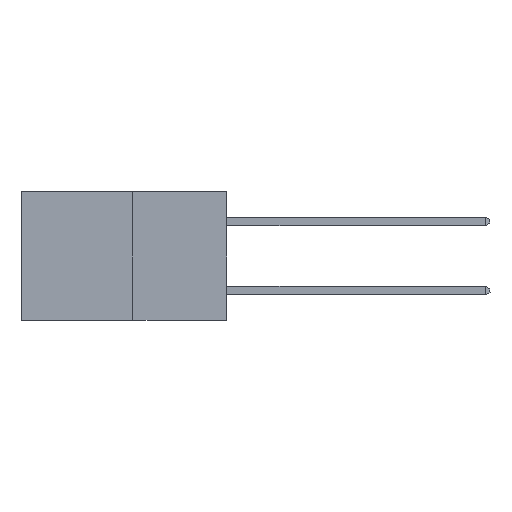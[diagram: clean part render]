
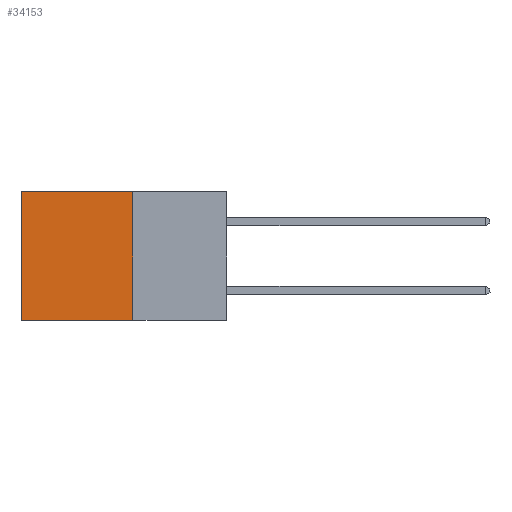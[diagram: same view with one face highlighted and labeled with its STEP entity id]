
A CAD part, left-side view. The second image highlights one B-rep face of the part: STEP entity #34153.
In plain terms, the highlighted planar face has unit normal (-1, 0, 0).
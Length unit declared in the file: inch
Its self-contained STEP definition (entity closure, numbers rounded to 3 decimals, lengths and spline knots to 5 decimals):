
#770 = VECTOR ( 'NONE', #28179, 39.37008 ) ;
#1699 = CARTESIAN_POINT ( 'NONE',  ( 0.277, 0.27, -0.37 ) ) ;
#2202 = DIRECTION ( 'NONE',  ( 0., 0., -1. ) ) ;
#2756 = VECTOR ( 'NONE', #32876, 39.37008 ) ;
#4413 = DIRECTION ( 'NONE',  ( 0., 1., 0. ) ) ;
#4956 = CARTESIAN_POINT ( 'NONE',  ( 0.277, 0.59, -0.37 ) ) ;
#6590 = EDGE_CURVE ( 'NONE', #33400, #20237, #7271, .T. ) ;
#7271 = LINE ( 'NONE', #12249, #770 ) ;
#7286 = ORIENTED_EDGE ( 'NONE', *, *, #25435, .T. ) ;
#8926 = CARTESIAN_POINT ( 'NONE',  ( 0.277, 0.27, 0. ) ) ;
#9166 = ORIENTED_EDGE ( 'NONE', *, *, #9793, .T. ) ;
#9630 = ORIENTED_EDGE ( 'NONE', *, *, #14568, .F. ) ;
#9793 = EDGE_CURVE ( 'NONE', #33400, #19299, #24046, .T. ) ;
#12108 = EDGE_LOOP ( 'NONE', ( #7286, #9630, #16774, #9166 ) ) ;
#12244 = CARTESIAN_POINT ( 'NONE',  ( 0.277, 0.27, -0.37 ) ) ;
#12249 = CARTESIAN_POINT ( 'NONE',  ( 0.277, 0.27, -0.37 ) ) ;
#14568 = EDGE_CURVE ( 'NONE', #20237, #20896, #26388, .T. ) ;
#14912 = DIRECTION ( 'NONE',  ( 0., 0., -1. ) ) ;
#15228 = VECTOR ( 'NONE', #2202, 39.37008 ) ;
#16545 = FACE_OUTER_BOUND ( 'NONE', #12108, .T. ) ;
#16774 = ORIENTED_EDGE ( 'NONE', *, *, #6590, .F. ) ;
#18245 = CARTESIAN_POINT ( 'NONE',  ( 0.277, 0.59, -0.37 ) ) ;
#19097 = AXIS2_PLACEMENT_3D ( 'NONE', #12244, #30881, #14912 ) ;
#19299 = VERTEX_POINT ( 'NONE', #20249 ) ;
#19492 = CARTESIAN_POINT ( 'NONE',  ( 0.277, 0.27, 0. ) ) ;
#20237 = VERTEX_POINT ( 'NONE', #34426 ) ;
#20249 = CARTESIAN_POINT ( 'NONE',  ( 0.277, 0.59, 0. ) ) ;
#20896 = VERTEX_POINT ( 'NONE', #4956 ) ;
#24046 = LINE ( 'NONE', #8926, #2756 ) ;
#25435 = EDGE_CURVE ( 'NONE', #19299, #20896, #28561, .T. ) ;
#25500 = PLANE ( 'NONE',  #19097 ) ;
#26388 = LINE ( 'NONE', #1699, #32613 ) ;
#28179 = DIRECTION ( 'NONE',  ( 0., 0., -1. ) ) ;
#28561 = LINE ( 'NONE', #18245, #15228 ) ;
#30881 = DIRECTION ( 'NONE',  ( 1., 0., 0. ) ) ;
#32613 = VECTOR ( 'NONE', #4413, 39.37008 ) ;
#32876 = DIRECTION ( 'NONE',  ( 0., 1., 0. ) ) ;
#33400 = VERTEX_POINT ( 'NONE', #19492 ) ;
#34153 = ADVANCED_FACE ( 'NONE', ( #16545 ), #25500, .F. ) ;
#34426 = CARTESIAN_POINT ( 'NONE',  ( 0.277, 0.27, -0.37 ) ) ;
